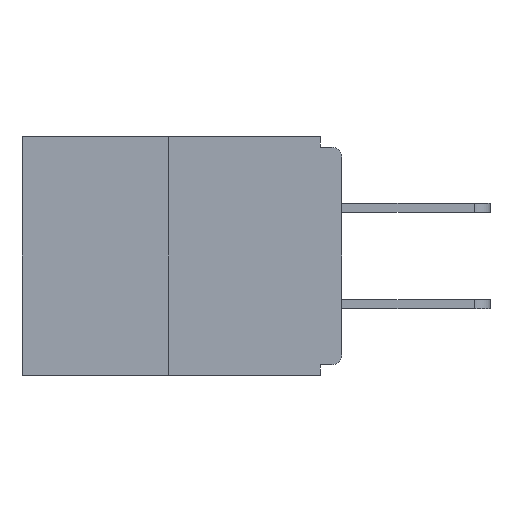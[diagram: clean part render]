
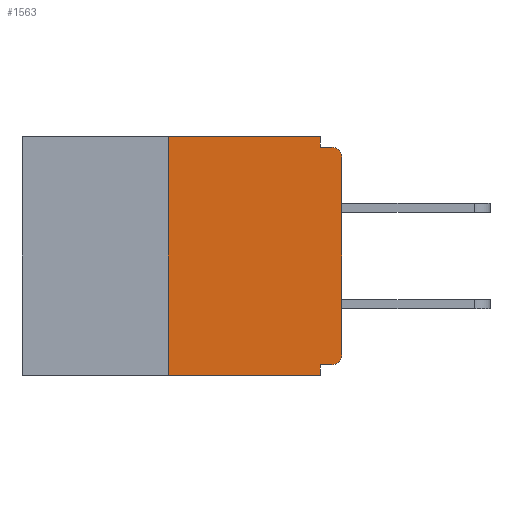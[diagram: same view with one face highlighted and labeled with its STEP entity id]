
A CAD part, left-side view. The second image highlights one B-rep face of the part: STEP entity #1563.
In plain terms, the highlighted planar face has unit normal (-1, 0, 0).
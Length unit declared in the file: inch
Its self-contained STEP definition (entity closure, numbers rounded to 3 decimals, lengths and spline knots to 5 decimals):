
#786 = VERTEX_POINT ( 'NONE', #12403 ) ;
#808 = VERTEX_POINT ( 'NONE', #11154 ) ;
#990 = CARTESIAN_POINT ( 'NONE',  ( 0., 0.031, -0.343 ) ) ;
#1152 = CARTESIAN_POINT ( 'NONE',  ( 0., 0.46, 0. ) ) ;
#1227 = LINE ( 'NONE', #990, #11766 ) ;
#1255 = VERTEX_POINT ( 'NONE', #13041 ) ;
#1563 = ADVANCED_FACE ( 'NONE', ( #13132 ), #15286, .F. ) ;
#1804 = CARTESIAN_POINT ( 'NONE',  ( 0., 0.46, -0.343 ) ) ;
#1834 = CARTESIAN_POINT ( 'NONE',  ( 0., 0.015, -0.313 ) ) ;
#2389 = CARTESIAN_POINT ( 'NONE',  ( 0., 0., -0.328 ) ) ;
#2420 = LINE ( 'NONE', #16424, #3421 ) ;
#3342 = CARTESIAN_POINT ( 'NONE',  ( 0., 0.015, -0.03 ) ) ;
#3421 = VECTOR ( 'NONE', #9770, 39.37008 ) ;
#3434 = EDGE_CURVE ( 'NONE', #3955, #4102, #4911, .T. ) ;
#3484 = VERTEX_POINT ( 'NONE', #8905 ) ;
#3661 = EDGE_CURVE ( 'NONE', #5301, #808, #16260, .T. ) ;
#3955 = VERTEX_POINT ( 'NONE', #13328 ) ;
#3988 = ORIENTED_EDGE ( 'NONE', *, *, #14646, .T. ) ;
#3989 = DIRECTION ( 'NONE',  ( 0., 0., 1. ) ) ;
#3993 = LINE ( 'NONE', #13625, #16149 ) ;
#4102 = VERTEX_POINT ( 'NONE', #14259 ) ;
#4335 = DIRECTION ( 'NONE',  ( 0., 0., 1. ) ) ;
#4388 = ORIENTED_EDGE ( 'NONE', *, *, #11538, .T. ) ;
#4646 = DIRECTION ( 'NONE',  ( -1., 0., 0. ) ) ;
#4792 = VERTEX_POINT ( 'NONE', #10938 ) ;
#4911 = LINE ( 'NONE', #2389, #6117 ) ;
#5301 = VERTEX_POINT ( 'NONE', #13992 ) ;
#5602 = AXIS2_PLACEMENT_3D ( 'NONE', #1834, #9587, #13498 ) ;
#5621 = DIRECTION ( 'NONE',  ( 0., 0., -1. ) ) ;
#6117 = VECTOR ( 'NONE', #13943, 39.37008 ) ;
#6687 = CARTESIAN_POINT ( 'NONE',  ( 0., 0.46, 0. ) ) ;
#6890 = EDGE_CURVE ( 'NONE', #1255, #4792, #14221, .T. ) ;
#6914 = CARTESIAN_POINT ( 'NONE',  ( 0., 0.015, -0.015 ) ) ;
#6991 = CIRCLE ( 'NONE', #11385, 0.015 ) ;
#7035 = DIRECTION ( 'NONE',  ( 0., -1., 0. ) ) ;
#7279 = DIRECTION ( 'NONE',  ( 0., 0., -1. ) ) ;
#7539 = ORIENTED_EDGE ( 'NONE', *, *, #8934, .F. ) ;
#7760 = ORIENTED_EDGE ( 'NONE', *, *, #6890, .T. ) ;
#8004 = DIRECTION ( 'NONE',  ( 0., -1., 0. ) ) ;
#8019 = VECTOR ( 'NONE', #3989, 39.37008 ) ;
#8258 = ORIENTED_EDGE ( 'NONE', *, *, #3434, .F. ) ;
#8790 = DIRECTION ( 'NONE',  ( 0., 0., -1. ) ) ;
#8840 = DIRECTION ( 'NONE',  ( 1., 0., 0. ) ) ;
#8905 = CARTESIAN_POINT ( 'NONE',  ( 0., 0., -0.313 ) ) ;
#8934 = EDGE_CURVE ( 'NONE', #808, #10004, #2420, .T. ) ;
#8964 = VECTOR ( 'NONE', #7035, 39.37008 ) ;
#9587 = DIRECTION ( 'NONE',  ( -1., 0., 0. ) ) ;
#9691 = EDGE_CURVE ( 'NONE', #11996, #10004, #6991, .T. ) ;
#9770 = DIRECTION ( 'NONE',  ( 0., -1., 0. ) ) ;
#9895 = CARTESIAN_POINT ( 'NONE',  ( 0., 0., -0.03 ) ) ;
#10004 = VERTEX_POINT ( 'NONE', #6914 ) ;
#10170 = ORIENTED_EDGE ( 'NONE', *, *, #14489, .F. ) ;
#10352 = CIRCLE ( 'NONE', #5602, 0.015 ) ;
#10382 = CARTESIAN_POINT ( 'NONE',  ( 0., 0., 0. ) ) ;
#10526 = CARTESIAN_POINT ( 'NONE',  ( 0., 0.031, 0. ) ) ;
#10938 = CARTESIAN_POINT ( 'NONE',  ( 0., 0.031, -0.343 ) ) ;
#11113 = LINE ( 'NONE', #6687, #12111 ) ;
#11154 = CARTESIAN_POINT ( 'NONE',  ( 0., 0.031, -0.015 ) ) ;
#11385 = AXIS2_PLACEMENT_3D ( 'NONE', #3342, #4646, #7279 ) ;
#11538 = EDGE_CURVE ( 'NONE', #3955, #3484, #10352, .T. ) ;
#11717 = EDGE_LOOP ( 'NONE', ( #16441, #10170, #7760, #15930, #8258, #4388, #3988, #12049, #7539, #14642 ) ) ;
#11766 = VECTOR ( 'NONE', #8790, 39.37008 ) ;
#11996 = VERTEX_POINT ( 'NONE', #9895 ) ;
#12049 = ORIENTED_EDGE ( 'NONE', *, *, #9691, .T. ) ;
#12111 = VECTOR ( 'NONE', #8004, 39.37008 ) ;
#12403 = CARTESIAN_POINT ( 'NONE',  ( 0., 0.25, 0. ) ) ;
#12996 = EDGE_CURVE ( 'NONE', #4102, #4792, #1227, .T. ) ;
#13041 = CARTESIAN_POINT ( 'NONE',  ( 0., 0.25, -0.343 ) ) ;
#13132 = FACE_OUTER_BOUND ( 'NONE', #11717, .T. ) ;
#13328 = CARTESIAN_POINT ( 'NONE',  ( 0., 0.015, -0.328 ) ) ;
#13498 = DIRECTION ( 'NONE',  ( 0., 0., -1. ) ) ;
#13625 = CARTESIAN_POINT ( 'NONE',  ( 0., 0.25, 0. ) ) ;
#13943 = DIRECTION ( 'NONE',  ( 0., 1., 0. ) ) ;
#13992 = CARTESIAN_POINT ( 'NONE',  ( 0., 0.031, 0. ) ) ;
#14221 = LINE ( 'NONE', #1804, #8964 ) ;
#14230 = VECTOR ( 'NONE', #5621, 39.37008 ) ;
#14259 = CARTESIAN_POINT ( 'NONE',  ( 0., 0.031, -0.328 ) ) ;
#14268 = EDGE_CURVE ( 'NONE', #786, #5301, #11113, .T. ) ;
#14489 = EDGE_CURVE ( 'NONE', #1255, #786, #3993, .T. ) ;
#14642 = ORIENTED_EDGE ( 'NONE', *, *, #3661, .F. ) ;
#14646 = EDGE_CURVE ( 'NONE', #3484, #11996, #15335, .T. ) ;
#14714 = AXIS2_PLACEMENT_3D ( 'NONE', #1152, #8840, #15345 ) ;
#15286 = PLANE ( 'NONE',  #14714 ) ;
#15335 = LINE ( 'NONE', #10382, #8019 ) ;
#15345 = DIRECTION ( 'NONE',  ( 0., 0., -1. ) ) ;
#15930 = ORIENTED_EDGE ( 'NONE', *, *, #12996, .F. ) ;
#16149 = VECTOR ( 'NONE', #4335, 39.37008 ) ;
#16260 = LINE ( 'NONE', #10526, #14230 ) ;
#16424 = CARTESIAN_POINT ( 'NONE',  ( 0., 0., -0.015 ) ) ;
#16441 = ORIENTED_EDGE ( 'NONE', *, *, #14268, .F. ) ;
